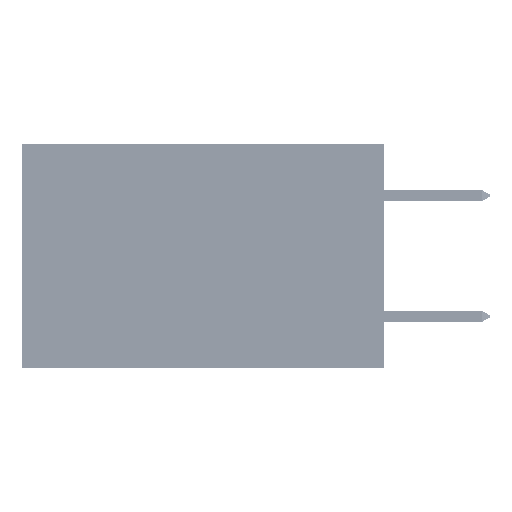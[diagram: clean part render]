
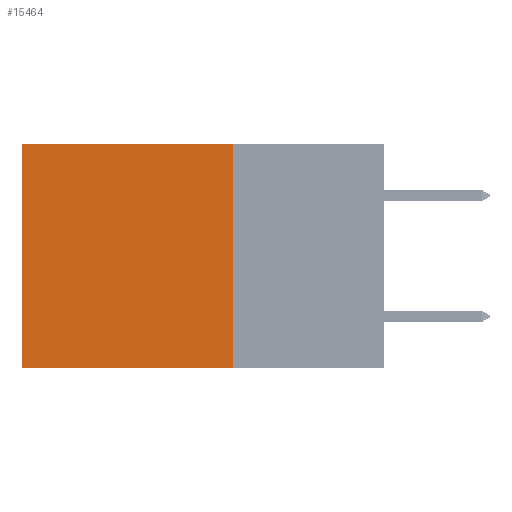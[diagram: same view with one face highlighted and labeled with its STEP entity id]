
A CAD part, left-side view. The second image highlights one B-rep face of the part: STEP entity #15464.
In plain terms, the highlighted planar face has unit normal (-1, 0, 0).
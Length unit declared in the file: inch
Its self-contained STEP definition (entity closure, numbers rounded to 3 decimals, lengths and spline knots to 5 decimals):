
#509 = CARTESIAN_POINT ( 'NONE',  ( 0.2875, 0.25, 0. ) ) ;
#1432 = LINE ( 'NONE', #42661, #26674 ) ;
#4138 = VERTEX_POINT ( 'NONE', #47893 ) ;
#4298 = ORIENTED_EDGE ( 'NONE', *, *, #34562, .F. ) ;
#4851 = CARTESIAN_POINT ( 'NONE',  ( 0.2875, 0.6, -0.37 ) ) ;
#5572 = EDGE_CURVE ( 'NONE', #4138, #5673, #34156, .T. ) ;
#5673 = VERTEX_POINT ( 'NONE', #30694 ) ;
#6133 = PLANE ( 'NONE',  #11838 ) ;
#6379 = DIRECTION ( 'NONE',  ( 0., 0., -1. ) ) ;
#8115 = LINE ( 'NONE', #509, #16018 ) ;
#10569 = FACE_OUTER_BOUND ( 'NONE', #22411, .T. ) ;
#10801 = CARTESIAN_POINT ( 'NONE',  ( 0.2875, 0.25, 0. ) ) ;
#11113 = LINE ( 'NONE', #30213, #47224 ) ;
#11838 = AXIS2_PLACEMENT_3D ( 'NONE', #10801, #25770, #6379 ) ;
#15464 = ADVANCED_FACE ( 'NONE', ( #10569 ), #6133, .F. ) ;
#16018 = VECTOR ( 'NONE', #38271, 39.37008 ) ;
#19402 = VERTEX_POINT ( 'NONE', #4851 ) ;
#21869 = ORIENTED_EDGE ( 'NONE', *, *, #37436, .T. ) ;
#22411 = EDGE_LOOP ( 'NONE', ( #21869, #4298, #25593, #44007 ) ) ;
#25593 = ORIENTED_EDGE ( 'NONE', *, *, #26062, .F. ) ;
#25770 = DIRECTION ( 'NONE',  ( 1., 0., 0. ) ) ;
#26062 = EDGE_CURVE ( 'NONE', #4138, #27556, #8115, .T. ) ;
#26674 = VECTOR ( 'NONE', #43149, 39.37008 ) ;
#27556 = VERTEX_POINT ( 'NONE', #43168 ) ;
#30213 = CARTESIAN_POINT ( 'NONE',  ( 0.2875, 0.6, 0. ) ) ;
#30694 = CARTESIAN_POINT ( 'NONE',  ( 0.2875, 0.6, 0. ) ) ;
#34156 = LINE ( 'NONE', #41271, #35580 ) ;
#34562 = EDGE_CURVE ( 'NONE', #27556, #19402, #1432, .T. ) ;
#35580 = VECTOR ( 'NONE', #38522, 39.37008 ) ;
#37333 = DIRECTION ( 'NONE',  ( 0., 0., -1. ) ) ;
#37436 = EDGE_CURVE ( 'NONE', #5673, #19402, #11113, .T. ) ;
#38271 = DIRECTION ( 'NONE',  ( 0., 0., -1. ) ) ;
#38522 = DIRECTION ( 'NONE',  ( 0., 1., 0. ) ) ;
#41271 = CARTESIAN_POINT ( 'NONE',  ( 0.2875, 0.25, 0. ) ) ;
#42661 = CARTESIAN_POINT ( 'NONE',  ( 0.2875, 0.25, -0.37 ) ) ;
#43149 = DIRECTION ( 'NONE',  ( 0., 1., 0. ) ) ;
#43168 = CARTESIAN_POINT ( 'NONE',  ( 0.2875, 0.25, -0.37 ) ) ;
#44007 = ORIENTED_EDGE ( 'NONE', *, *, #5572, .T. ) ;
#47224 = VECTOR ( 'NONE', #37333, 39.37008 ) ;
#47893 = CARTESIAN_POINT ( 'NONE',  ( 0.2875, 0.25, 0. ) ) ;
